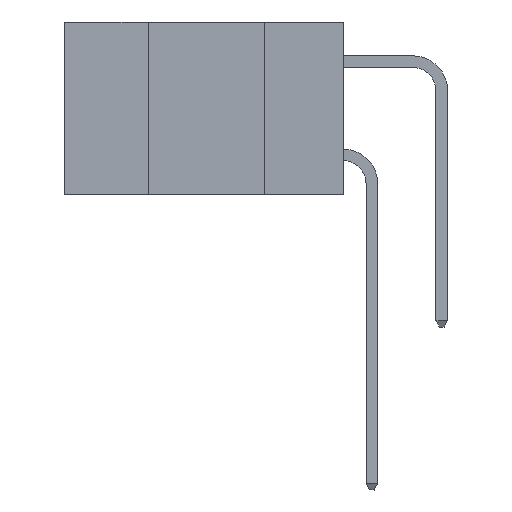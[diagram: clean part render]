
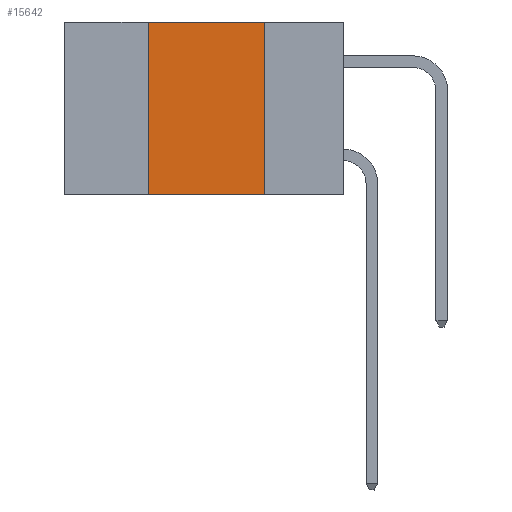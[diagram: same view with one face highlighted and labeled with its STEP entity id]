
A CAD part, left-side view. The second image highlights one B-rep face of the part: STEP entity #15642.
In plain terms, the highlighted planar face has unit normal (-1, 0, 0).
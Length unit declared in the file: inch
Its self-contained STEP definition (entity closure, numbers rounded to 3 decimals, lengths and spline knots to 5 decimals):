
#408 = EDGE_CURVE ( 'NONE', #19645, #6066, #14465, .T. ) ;
#872 = EDGE_LOOP ( 'NONE', ( #16024, #4935, #8365, #7272 ) ) ;
#940 = DIRECTION ( 'NONE',  ( 0., -1., 0. ) ) ;
#1040 = LINE ( 'NONE', #16923, #1720 ) ;
#1720 = VECTOR ( 'NONE', #940, 39.37008 ) ;
#2431 = EDGE_CURVE ( 'NONE', #12329, #6066, #13298, .T. ) ;
#2706 = CARTESIAN_POINT ( 'NONE',  ( 0., 0.42, -0.37 ) ) ;
#3440 = AXIS2_PLACEMENT_3D ( 'NONE', #4044, #8861, #15293 ) ;
#3715 = VERTEX_POINT ( 'NONE', #20455 ) ;
#4044 = CARTESIAN_POINT ( 'NONE',  ( 0., 0.6, 0. ) ) ;
#4165 = CARTESIAN_POINT ( 'NONE',  ( 0., 0.42, -0.37 ) ) ;
#4935 = ORIENTED_EDGE ( 'NONE', *, *, #17738, .F. ) ;
#6066 = VERTEX_POINT ( 'NONE', #14116 ) ;
#6157 = DIRECTION ( 'NONE',  ( 0., 0., -1. ) ) ;
#7272 = ORIENTED_EDGE ( 'NONE', *, *, #2431, .T. ) ;
#8365 = ORIENTED_EDGE ( 'NONE', *, *, #20033, .F. ) ;
#8861 = DIRECTION ( 'NONE',  ( 1., 0., 0. ) ) ;
#10697 = CARTESIAN_POINT ( 'NONE',  ( 0., 0.17, 0. ) ) ;
#11347 = VECTOR ( 'NONE', #6157, 39.37008 ) ;
#11787 = VECTOR ( 'NONE', #15199, 39.37008 ) ;
#12025 = FACE_OUTER_BOUND ( 'NONE', #872, .T. ) ;
#12329 = VERTEX_POINT ( 'NONE', #2706 ) ;
#13298 = LINE ( 'NONE', #19495, #17246 ) ;
#13624 = LINE ( 'NONE', #4165, #11787 ) ;
#14116 = CARTESIAN_POINT ( 'NONE',  ( 0., 0.17, -0.37 ) ) ;
#14465 = LINE ( 'NONE', #16041, #11347 ) ;
#14749 = DIRECTION ( 'NONE',  ( 0., -1., 0. ) ) ;
#15199 = DIRECTION ( 'NONE',  ( 0., 0., 1. ) ) ;
#15293 = DIRECTION ( 'NONE',  ( 0., 0., -1. ) ) ;
#15642 = ADVANCED_FACE ( 'NONE', ( #12025 ), #18464, .F. ) ;
#16024 = ORIENTED_EDGE ( 'NONE', *, *, #408, .F. ) ;
#16041 = CARTESIAN_POINT ( 'NONE',  ( 0., 0.17, -0.37 ) ) ;
#16923 = CARTESIAN_POINT ( 'NONE',  ( 0., 0.6, 0. ) ) ;
#17246 = VECTOR ( 'NONE', #14749, 39.37008 ) ;
#17738 = EDGE_CURVE ( 'NONE', #3715, #19645, #1040, .T. ) ;
#18464 = PLANE ( 'NONE',  #3440 ) ;
#19495 = CARTESIAN_POINT ( 'NONE',  ( 0., 0.6, -0.37 ) ) ;
#19645 = VERTEX_POINT ( 'NONE', #10697 ) ;
#20033 = EDGE_CURVE ( 'NONE', #12329, #3715, #13624, .T. ) ;
#20455 = CARTESIAN_POINT ( 'NONE',  ( 0., 0.42, 0. ) ) ;
